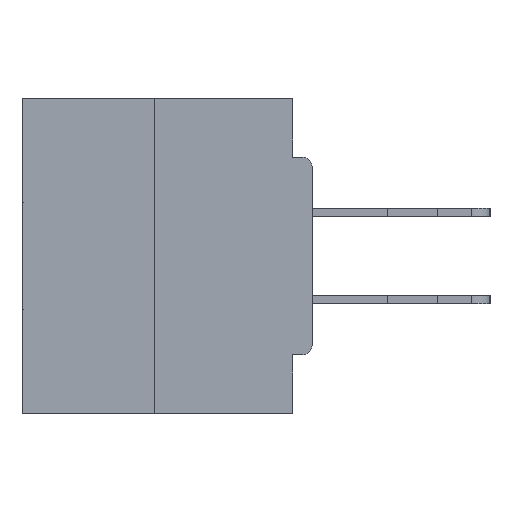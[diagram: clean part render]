
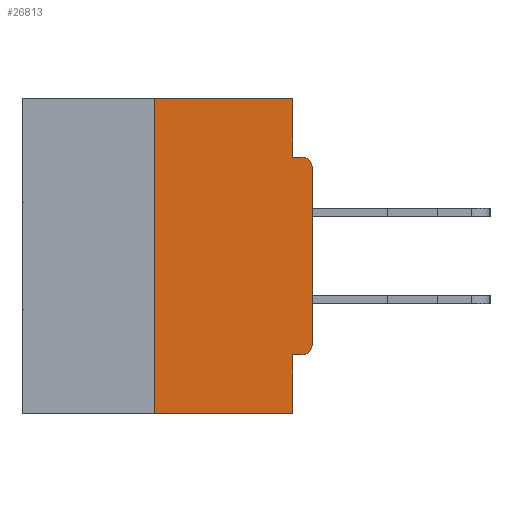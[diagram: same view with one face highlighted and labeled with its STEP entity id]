
A CAD part, left-side view. The second image highlights one B-rep face of the part: STEP entity #26813.
In plain terms, the highlighted planar face has unit normal (-1, 0, 0).
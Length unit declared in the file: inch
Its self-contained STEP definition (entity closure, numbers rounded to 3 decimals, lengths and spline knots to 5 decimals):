
#375 = CARTESIAN_POINT ( 'NONE',  ( 0., 0., -0.4065 ) ) ;
#479 = CARTESIAN_POINT ( 'NONE',  ( 0., 0.015, -0.1085 ) ) ;
#537 = VERTEX_POINT ( 'NONE', #29293 ) ;
#1288 = DIRECTION ( 'NONE',  ( 0., 0., -1. ) ) ;
#2445 = VERTEX_POINT ( 'NONE', #16595 ) ;
#2856 = ORIENTED_EDGE ( 'NONE', *, *, #37111, .T. ) ;
#3335 = EDGE_CURVE ( 'NONE', #7968, #36847, #20007, .T. ) ;
#3617 = DIRECTION ( 'NONE',  ( 0., -1., 0. ) ) ;
#4344 = DIRECTION ( 'NONE',  ( -1., 0., 0. ) ) ;
#4995 = ORIENTED_EDGE ( 'NONE', *, *, #9207, .F. ) ;
#5865 = PLANE ( 'NONE',  #10245 ) ;
#6116 = CARTESIAN_POINT ( 'NONE',  ( 0., 0.46, -0.5 ) ) ;
#6302 = CARTESIAN_POINT ( 'NONE',  ( 0., 0.015, -0.0935 ) ) ;
#6545 = CARTESIAN_POINT ( 'NONE',  ( 0., 0.25, 0. ) ) ;
#6754 = ORIENTED_EDGE ( 'NONE', *, *, #35620, .T. ) ;
#6821 = DIRECTION ( 'NONE',  ( 0., 0., 1. ) ) ;
#7968 = VERTEX_POINT ( 'NONE', #37014 ) ;
#8211 = DIRECTION ( 'NONE',  ( 0., 0., -1. ) ) ;
#9207 = EDGE_CURVE ( 'NONE', #21637, #15661, #16882, .T. ) ;
#9447 = CARTESIAN_POINT ( 'NONE',  ( 0., 0.25, -0.5 ) ) ;
#10245 = AXIS2_PLACEMENT_3D ( 'NONE', #31399, #12092, #28081 ) ;
#10990 = ORIENTED_EDGE ( 'NONE', *, *, #30663, .F. ) ;
#11164 = DIRECTION ( 'NONE',  ( 0., 0., 1. ) ) ;
#11218 = VECTOR ( 'NONE', #6821, 39.37008 ) ;
#12092 = DIRECTION ( 'NONE',  ( 1., 0., 0. ) ) ;
#12890 = EDGE_CURVE ( 'NONE', #2445, #39000, #26700, .T. ) ;
#14147 = CARTESIAN_POINT ( 'NONE',  ( 0., 0.015, -0.3915 ) ) ;
#14735 = EDGE_CURVE ( 'NONE', #29829, #21637, #39400, .T. ) ;
#15621 = EDGE_CURVE ( 'NONE', #26888, #29829, #35879, .T. ) ;
#15661 = VERTEX_POINT ( 'NONE', #39078 ) ;
#15710 = ORIENTED_EDGE ( 'NONE', *, *, #12890, .F. ) ;
#16254 = ORIENTED_EDGE ( 'NONE', *, *, #35132, .T. ) ;
#16311 = VECTOR ( 'NONE', #36005, 39.37008 ) ;
#16595 = CARTESIAN_POINT ( 'NONE',  ( 0., 0.015, -0.4065 ) ) ;
#16882 = LINE ( 'NONE', #30126, #19869 ) ;
#18778 = AXIS2_PLACEMENT_3D ( 'NONE', #479, #4344, #39374 ) ;
#18779 = LINE ( 'NONE', #33211, #16311 ) ;
#18977 = VECTOR ( 'NONE', #11164, 39.37008 ) ;
#19208 = CARTESIAN_POINT ( 'NONE',  ( 0., 0.46, 0. ) ) ;
#19869 = VECTOR ( 'NONE', #31829, 39.37008 ) ;
#20007 = CIRCLE ( 'NONE', #18778, 0.015 ) ;
#20865 = ORIENTED_EDGE ( 'NONE', *, *, #3335, .T. ) ;
#21637 = VERTEX_POINT ( 'NONE', #35793 ) ;
#22131 = DIRECTION ( 'NONE',  ( 0., -1., 0. ) ) ;
#23095 = ORIENTED_EDGE ( 'NONE', *, *, #15621, .F. ) ;
#23278 = CIRCLE ( 'NONE', #34380, 0.015 ) ;
#23941 = DIRECTION ( 'NONE',  ( -1., 0., 0. ) ) ;
#24730 = VECTOR ( 'NONE', #32252, 39.37008 ) ;
#26700 = LINE ( 'NONE', #375, #24730 ) ;
#26813 = ADVANCED_FACE ( 'NONE', ( #38355 ), #5865, .F. ) ;
#26888 = VERTEX_POINT ( 'NONE', #9447 ) ;
#27101 = CARTESIAN_POINT ( 'NONE',  ( 0., 0.031, -0.5 ) ) ;
#27861 = CARTESIAN_POINT ( 'NONE',  ( 0., 0., -0.3915 ) ) ;
#28081 = DIRECTION ( 'NONE',  ( 0., 0., -1. ) ) ;
#29293 = CARTESIAN_POINT ( 'NONE',  ( 0., 0.031, -0.5 ) ) ;
#29352 = LINE ( 'NONE', #30010, #18977 ) ;
#29829 = VERTEX_POINT ( 'NONE', #30283 ) ;
#30010 = CARTESIAN_POINT ( 'NONE',  ( 0., 0., 0. ) ) ;
#30126 = CARTESIAN_POINT ( 'NONE',  ( 0., 0.031, 0. ) ) ;
#30283 = CARTESIAN_POINT ( 'NONE',  ( 0., 0.25, 0. ) ) ;
#30646 = VECTOR ( 'NONE', #8211, 39.37008 ) ;
#30663 = EDGE_CURVE ( 'NONE', #15661, #36847, #18779, .T. ) ;
#31399 = CARTESIAN_POINT ( 'NONE',  ( 0., 0.46, 0. ) ) ;
#31829 = DIRECTION ( 'NONE',  ( 0., 0., -1. ) ) ;
#32218 = ORIENTED_EDGE ( 'NONE', *, *, #37077, .F. ) ;
#32252 = DIRECTION ( 'NONE',  ( 0., 1., 0. ) ) ;
#33211 = CARTESIAN_POINT ( 'NONE',  ( 0., 0., -0.0935 ) ) ;
#33693 = ORIENTED_EDGE ( 'NONE', *, *, #14735, .F. ) ;
#33722 = LINE ( 'NONE', #6116, #35728 ) ;
#34380 = AXIS2_PLACEMENT_3D ( 'NONE', #14147, #23941, #1288 ) ;
#35132 = EDGE_CURVE ( 'NONE', #40376, #7968, #29352, .T. ) ;
#35620 = EDGE_CURVE ( 'NONE', #26888, #537, #33722, .T. ) ;
#35728 = VECTOR ( 'NONE', #22131, 39.37008 ) ;
#35793 = CARTESIAN_POINT ( 'NONE',  ( 0., 0.031, 0. ) ) ;
#35879 = LINE ( 'NONE', #6545, #11218 ) ;
#36005 = DIRECTION ( 'NONE',  ( 0., -1., 0. ) ) ;
#36847 = VERTEX_POINT ( 'NONE', #6302 ) ;
#36873 = EDGE_LOOP ( 'NONE', ( #33693, #23095, #6754, #32218, #15710, #2856, #16254, #20865, #10990, #4995 ) ) ;
#37014 = CARTESIAN_POINT ( 'NONE',  ( 0., 0., -0.1085 ) ) ;
#37077 = EDGE_CURVE ( 'NONE', #39000, #537, #39539, .T. ) ;
#37111 = EDGE_CURVE ( 'NONE', #2445, #40376, #23278, .T. ) ;
#38212 = CARTESIAN_POINT ( 'NONE',  ( 0., 0.031, -0.4065 ) ) ;
#38355 = FACE_OUTER_BOUND ( 'NONE', #36873, .T. ) ;
#38950 = VECTOR ( 'NONE', #3617, 39.37008 ) ;
#39000 = VERTEX_POINT ( 'NONE', #38212 ) ;
#39078 = CARTESIAN_POINT ( 'NONE',  ( 0., 0.031, -0.0935 ) ) ;
#39374 = DIRECTION ( 'NONE',  ( 0., 0., -1. ) ) ;
#39400 = LINE ( 'NONE', #19208, #38950 ) ;
#39539 = LINE ( 'NONE', #27101, #30646 ) ;
#40376 = VERTEX_POINT ( 'NONE', #27861 ) ;
